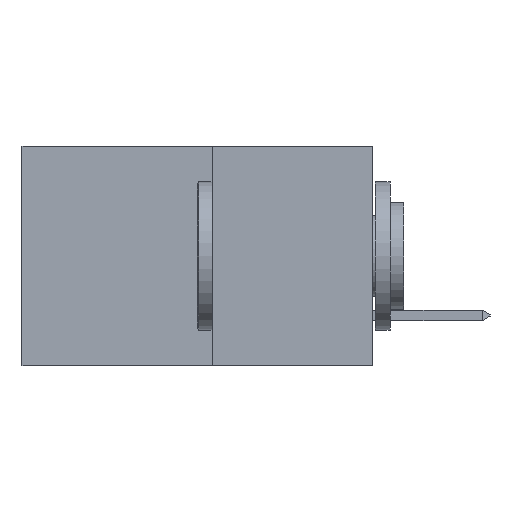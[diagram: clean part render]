
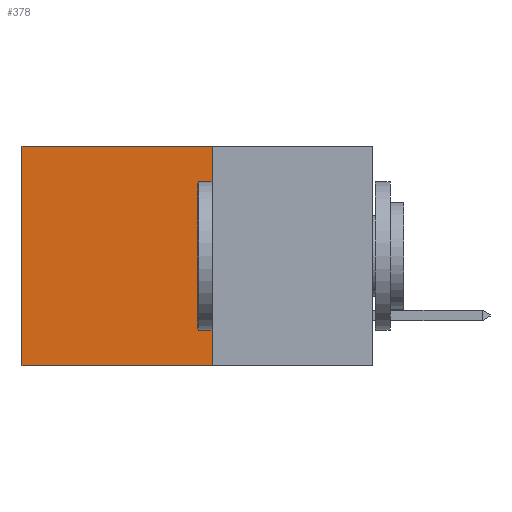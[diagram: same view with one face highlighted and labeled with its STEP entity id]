
A CAD part, left-side view. The second image highlights one B-rep face of the part: STEP entity #378.
In plain terms, the highlighted planar face has unit normal (-1, 0, 0).
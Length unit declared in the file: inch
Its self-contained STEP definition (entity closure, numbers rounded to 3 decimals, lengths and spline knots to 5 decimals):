
#117 = PLANE ( 'NONE',  #1835 ) ;
#378 = ADVANCED_FACE ( 'NONE', ( #8768 ), #117, .F. ) ;
#1002 = DIRECTION ( 'NONE',  ( 0., 0., -1. ) ) ;
#1046 = CARTESIAN_POINT ( 'NONE',  ( 0.277, 0.27, 0. ) ) ;
#1054 = ORIENTED_EDGE ( 'NONE', *, *, #6166, .T. ) ;
#1159 = EDGE_CURVE ( 'NONE', #4624, #12794, #10622, .T. ) ;
#1835 = AXIS2_PLACEMENT_3D ( 'NONE', #11301, #17408, #1002 ) ;
#2432 = VECTOR ( 'NONE', #4994, 39.37008 ) ;
#3655 = ORIENTED_EDGE ( 'NONE', *, *, #6118, .F. ) ;
#4624 = VERTEX_POINT ( 'NONE', #14926 ) ;
#4994 = DIRECTION ( 'NONE',  ( 0., 0., -1. ) ) ;
#5509 = CARTESIAN_POINT ( 'NONE',  ( 0.277, 0.27, -0.37 ) ) ;
#5962 = CARTESIAN_POINT ( 'NONE',  ( 0.277, 0.59, -0.37 ) ) ;
#6118 = EDGE_CURVE ( 'NONE', #8723, #12794, #17666, .T. ) ;
#6149 = VECTOR ( 'NONE', #7865, 39.37008 ) ;
#6166 = EDGE_CURVE ( 'NONE', #10877, #4624, #16747, .T. ) ;
#7865 = DIRECTION ( 'NONE',  ( 0., 0., -1. ) ) ;
#8723 = VERTEX_POINT ( 'NONE', #16188 ) ;
#8768 = FACE_OUTER_BOUND ( 'NONE', #16008, .T. ) ;
#9581 = LINE ( 'NONE', #14029, #2432 ) ;
#10065 = DIRECTION ( 'NONE',  ( 0., 1., 0. ) ) ;
#10622 = LINE ( 'NONE', #5962, #6149 ) ;
#10877 = VERTEX_POINT ( 'NONE', #12855 ) ;
#11301 = CARTESIAN_POINT ( 'NONE',  ( 0.277, 0.27, -0.37 ) ) ;
#12188 = ORIENTED_EDGE ( 'NONE', *, *, #18985, .F. ) ;
#12730 = VECTOR ( 'NONE', #13167, 39.37008 ) ;
#12794 = VERTEX_POINT ( 'NONE', #16616 ) ;
#12855 = CARTESIAN_POINT ( 'NONE',  ( 0.277, 0.27, 0. ) ) ;
#13167 = DIRECTION ( 'NONE',  ( 0., 1., 0. ) ) ;
#13679 = VECTOR ( 'NONE', #10065, 39.37008 ) ;
#14029 = CARTESIAN_POINT ( 'NONE',  ( 0.277, 0.27, -0.37 ) ) ;
#14926 = CARTESIAN_POINT ( 'NONE',  ( 0.277, 0.59, 0. ) ) ;
#15289 = ORIENTED_EDGE ( 'NONE', *, *, #1159, .T. ) ;
#16008 = EDGE_LOOP ( 'NONE', ( #15289, #3655, #12188, #1054 ) ) ;
#16188 = CARTESIAN_POINT ( 'NONE',  ( 0.277, 0.27, -0.37 ) ) ;
#16616 = CARTESIAN_POINT ( 'NONE',  ( 0.277, 0.59, -0.37 ) ) ;
#16747 = LINE ( 'NONE', #1046, #12730 ) ;
#17408 = DIRECTION ( 'NONE',  ( 1., 0., 0. ) ) ;
#17666 = LINE ( 'NONE', #5509, #13679 ) ;
#18985 = EDGE_CURVE ( 'NONE', #10877, #8723, #9581, .T. ) ;
